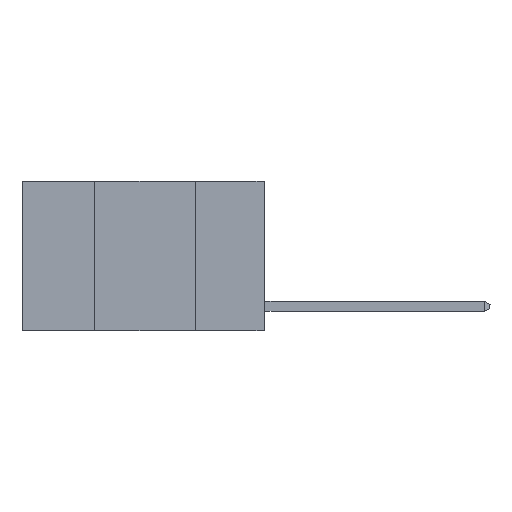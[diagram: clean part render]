
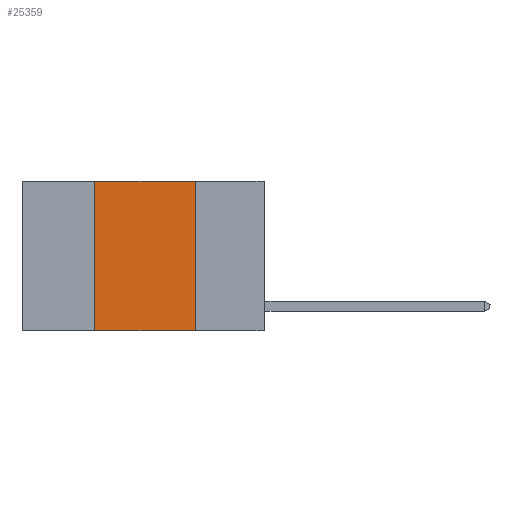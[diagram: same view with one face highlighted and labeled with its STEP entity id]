
A CAD part, left-side view. The second image highlights one B-rep face of the part: STEP entity #25359.
In plain terms, the highlighted planar face has unit normal (-1, 0, 0).
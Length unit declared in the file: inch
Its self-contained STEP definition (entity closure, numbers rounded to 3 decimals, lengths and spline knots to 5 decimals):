
#59 = EDGE_CURVE ( 'NONE', #11025, #21740, #14090, .T. ) ;
#334 = DIRECTION ( 'NONE',  ( 0., -1., 0. ) ) ;
#2585 = EDGE_CURVE ( 'NONE', #23574, #17846, #7935, .T. ) ;
#2984 = DIRECTION ( 'NONE',  ( 0., 0., 1. ) ) ;
#4269 = CARTESIAN_POINT ( 'NONE',  ( 0., 0.6, 0. ) ) ;
#5807 = EDGE_CURVE ( 'NONE', #23574, #21740, #8520, .T. ) ;
#7081 = CARTESIAN_POINT ( 'NONE',  ( 0., 0.17, 0. ) ) ;
#7091 = DIRECTION ( 'NONE',  ( 0., 0., -1. ) ) ;
#7189 = DIRECTION ( 'NONE',  ( 0., 0., -1. ) ) ;
#7935 = LINE ( 'NONE', #12765, #26100 ) ;
#8295 = VECTOR ( 'NONE', #7091, 39.37008 ) ;
#8325 = CARTESIAN_POINT ( 'NONE',  ( 0., 0.42, -0.37 ) ) ;
#8520 = LINE ( 'NONE', #11014, #21906 ) ;
#8834 = VECTOR ( 'NONE', #334, 39.37008 ) ;
#11014 = CARTESIAN_POINT ( 'NONE',  ( 0., 0.6, -0.37 ) ) ;
#11025 = VERTEX_POINT ( 'NONE', #7081 ) ;
#11561 = FACE_OUTER_BOUND ( 'NONE', #15915, .T. ) ;
#12108 = CARTESIAN_POINT ( 'NONE',  ( 0., 0.6, 0. ) ) ;
#12765 = CARTESIAN_POINT ( 'NONE',  ( 0., 0.42, 0. ) ) ;
#13985 = EDGE_CURVE ( 'NONE', #17846, #11025, #21370, .T. ) ;
#14090 = LINE ( 'NONE', #16276, #8295 ) ;
#14485 = CARTESIAN_POINT ( 'NONE',  ( 0., 0.42, 0. ) ) ;
#15257 = ORIENTED_EDGE ( 'NONE', *, *, #5807, .T. ) ;
#15360 = DIRECTION ( 'NONE',  ( 0., -1., 0. ) ) ;
#15915 = EDGE_LOOP ( 'NONE', ( #20333, #16164, #17428, #15257 ) ) ;
#16164 = ORIENTED_EDGE ( 'NONE', *, *, #13985, .F. ) ;
#16276 = CARTESIAN_POINT ( 'NONE',  ( 0., 0.17, 0. ) ) ;
#17428 = ORIENTED_EDGE ( 'NONE', *, *, #2585, .F. ) ;
#17846 = VERTEX_POINT ( 'NONE', #14485 ) ;
#18598 = CARTESIAN_POINT ( 'NONE',  ( 0., 0.17, -0.37 ) ) ;
#20069 = AXIS2_PLACEMENT_3D ( 'NONE', #4269, #21130, #7189 ) ;
#20333 = ORIENTED_EDGE ( 'NONE', *, *, #59, .F. ) ;
#20974 = PLANE ( 'NONE',  #20069 ) ;
#21130 = DIRECTION ( 'NONE',  ( 1., 0., 0. ) ) ;
#21370 = LINE ( 'NONE', #12108, #8834 ) ;
#21740 = VERTEX_POINT ( 'NONE', #18598 ) ;
#21906 = VECTOR ( 'NONE', #15360, 39.37008 ) ;
#23574 = VERTEX_POINT ( 'NONE', #8325 ) ;
#25359 = ADVANCED_FACE ( 'NONE', ( #11561 ), #20974, .F. ) ;
#26100 = VECTOR ( 'NONE', #2984, 39.37008 ) ;
